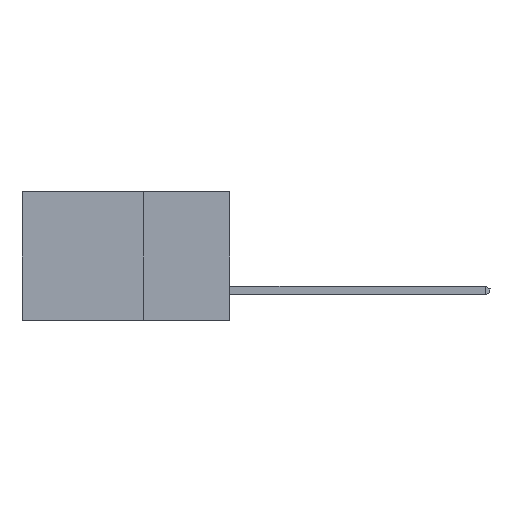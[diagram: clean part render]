
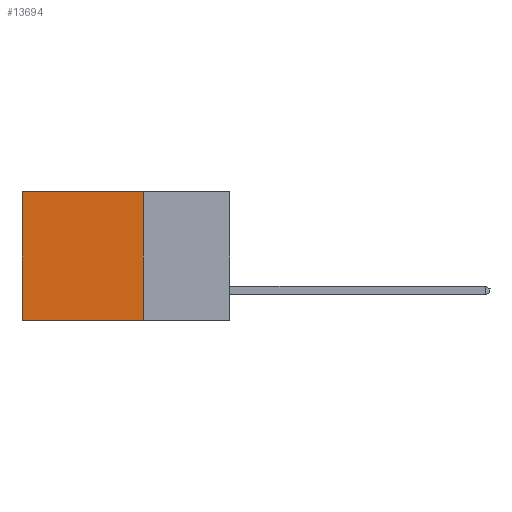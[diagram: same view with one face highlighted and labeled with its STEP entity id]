
A CAD part, left-side view. The second image highlights one B-rep face of the part: STEP entity #13694.
In plain terms, the highlighted planar face has unit normal (-1, 0, 0).
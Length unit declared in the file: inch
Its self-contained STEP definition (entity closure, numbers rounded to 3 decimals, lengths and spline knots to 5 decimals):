
#693 = CARTESIAN_POINT ( 'NONE',  ( 0.2615, 0.25, -0.37 ) ) ;
#951 = CARTESIAN_POINT ( 'NONE',  ( 0.2615, 0.25, -0.37 ) ) ;
#1141 = DIRECTION ( 'NONE',  ( 0., 1., 0. ) ) ;
#1453 = VERTEX_POINT ( 'NONE', #12467 ) ;
#1550 = EDGE_CURVE ( 'NONE', #12423, #5151, #15011, .T. ) ;
#1990 = CARTESIAN_POINT ( 'NONE',  ( 0.2615, 0.25, 0. ) ) ;
#2445 = EDGE_CURVE ( 'NONE', #1453, #12270, #8900, .T. ) ;
#2563 = EDGE_CURVE ( 'NONE', #5151, #12270, #3709, .T. ) ;
#2698 = VECTOR ( 'NONE', #4330, 39.37008 ) ;
#3709 = LINE ( 'NONE', #6968, #7791 ) ;
#4330 = DIRECTION ( 'NONE',  ( 0., 1., 0. ) ) ;
#4355 = FACE_OUTER_BOUND ( 'NONE', #10082, .T. ) ;
#4445 = CARTESIAN_POINT ( 'NONE',  ( 0.2615, 0.6, 0. ) ) ;
#5151 = VERTEX_POINT ( 'NONE', #4445 ) ;
#5350 = DIRECTION ( 'NONE',  ( 0., 0., -1. ) ) ;
#6429 = ORIENTED_EDGE ( 'NONE', *, *, #2445, .F. ) ;
#6968 = CARTESIAN_POINT ( 'NONE',  ( 0.2615, 0.6, -0.37 ) ) ;
#7731 = ORIENTED_EDGE ( 'NONE', *, *, #1550, .T. ) ;
#7791 = VECTOR ( 'NONE', #8352, 39.37008 ) ;
#8352 = DIRECTION ( 'NONE',  ( 0., 0., -1. ) ) ;
#8634 = ORIENTED_EDGE ( 'NONE', *, *, #2563, .T. ) ;
#8900 = LINE ( 'NONE', #951, #2698 ) ;
#8989 = CARTESIAN_POINT ( 'NONE',  ( 0.2615, 0.25, -0.37 ) ) ;
#9224 = ORIENTED_EDGE ( 'NONE', *, *, #10312, .F. ) ;
#10082 = EDGE_LOOP ( 'NONE', ( #8634, #6429, #9224, #7731 ) ) ;
#10312 = EDGE_CURVE ( 'NONE', #12423, #1453, #11157, .T. ) ;
#10720 = VECTOR ( 'NONE', #1141, 39.37008 ) ;
#11157 = LINE ( 'NONE', #693, #12632 ) ;
#11379 = DIRECTION ( 'NONE',  ( 1., 0., 0. ) ) ;
#11533 = CARTESIAN_POINT ( 'NONE',  ( 0.2615, 0.25, 0. ) ) ;
#12270 = VERTEX_POINT ( 'NONE', #12746 ) ;
#12384 = PLANE ( 'NONE',  #14448 ) ;
#12423 = VERTEX_POINT ( 'NONE', #1990 ) ;
#12467 = CARTESIAN_POINT ( 'NONE',  ( 0.2615, 0.25, -0.37 ) ) ;
#12632 = VECTOR ( 'NONE', #5350, 39.37008 ) ;
#12746 = CARTESIAN_POINT ( 'NONE',  ( 0.2615, 0.6, -0.37 ) ) ;
#13694 = ADVANCED_FACE ( 'NONE', ( #4355 ), #12384, .F. ) ;
#14448 = AXIS2_PLACEMENT_3D ( 'NONE', #8989, #11379, #14918 ) ;
#14918 = DIRECTION ( 'NONE',  ( 0., 0., -1. ) ) ;
#15011 = LINE ( 'NONE', #11533, #10720 ) ;
